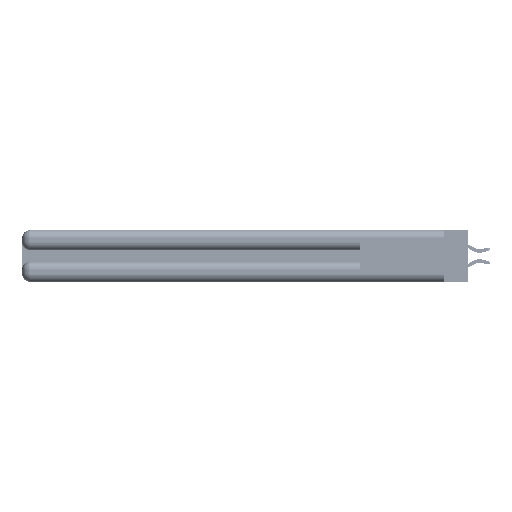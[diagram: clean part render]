
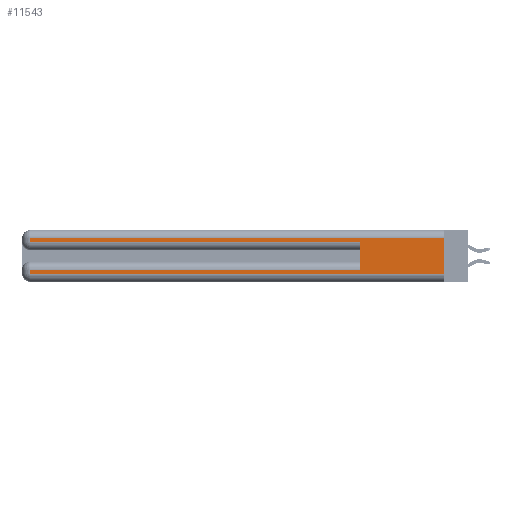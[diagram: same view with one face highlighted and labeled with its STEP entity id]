
A CAD part, left-side view. The second image highlights one B-rep face of the part: STEP entity #11543.
In plain terms, the highlighted planar face has unit normal (-1, 0, 0).
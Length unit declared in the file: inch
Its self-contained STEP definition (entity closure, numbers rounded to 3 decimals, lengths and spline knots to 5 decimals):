
#1251 = VERTEX_POINT ( 'NONE', #50723 ) ;
#2664 = ORIENTED_EDGE ( 'NONE', *, *, #31764, .T. ) ;
#2678 = CARTESIAN_POINT ( 'NONE',  ( 0., 2.94, 0.37 ) ) ;
#2749 = CARTESIAN_POINT ( 'NONE',  ( 0., 2.94, 0.06 ) ) ;
#3593 = LINE ( 'NONE', #9691, #13614 ) ;
#5487 = VECTOR ( 'NONE', #15396, 39.37008 ) ;
#5743 = VECTOR ( 'NONE', #54405, 39.37008 ) ;
#6292 = AXIS2_PLACEMENT_3D ( 'NONE', #16166, #46097, #20479 ) ;
#6643 = CARTESIAN_POINT ( 'NONE',  ( 0., 2.94, 0.31 ) ) ;
#7628 = PLANE ( 'NONE',  #6292 ) ;
#7849 = LINE ( 'NONE', #32007, #27851 ) ;
#8331 = CARTESIAN_POINT ( 'NONE',  ( 0., 0., 0.37 ) ) ;
#9218 = DIRECTION ( 'NONE',  ( 0., 1., 0. ) ) ;
#9309 = EDGE_CURVE ( 'NONE', #15465, #48542, #51947, .T. ) ;
#9337 = VECTOR ( 'NONE', #27100, 39.37008 ) ;
#9691 = CARTESIAN_POINT ( 'NONE',  ( 0., 0., 0.285 ) ) ;
#11543 = ADVANCED_FACE ( 'NONE', ( #34423 ), #7628, .F. ) ;
#12615 = CARTESIAN_POINT ( 'NONE',  ( 0., 0., 0.06 ) ) ;
#12629 = ORIENTED_EDGE ( 'NONE', *, *, #18950, .T. ) ;
#13614 = VECTOR ( 'NONE', #39954, 39.37008 ) ;
#13884 = VERTEX_POINT ( 'NONE', #6643 ) ;
#14214 = CARTESIAN_POINT ( 'NONE',  ( 0., 0., 0.31 ) ) ;
#15396 = DIRECTION ( 'NONE',  ( 0., 0., -1. ) ) ;
#15465 = VERTEX_POINT ( 'NONE', #48258 ) ;
#16166 = CARTESIAN_POINT ( 'NONE',  ( 0., 0., 0.37 ) ) ;
#16676 = ORIENTED_EDGE ( 'NONE', *, *, #44009, .T. ) ;
#17075 = LINE ( 'NONE', #45810, #5743 ) ;
#17283 = ORIENTED_EDGE ( 'NONE', *, *, #9309, .F. ) ;
#17862 = VECTOR ( 'NONE', #25252, 39.37008 ) ;
#18209 = EDGE_CURVE ( 'NONE', #24839, #1251, #7849, .T. ) ;
#18950 = EDGE_CURVE ( 'NONE', #13884, #49784, #17075, .T. ) ;
#20479 = DIRECTION ( 'NONE',  ( 0., 0., -1. ) ) ;
#23707 = CARTESIAN_POINT ( 'NONE',  ( 0., 2.94, 0.085 ) ) ;
#24839 = VERTEX_POINT ( 'NONE', #25220 ) ;
#24963 = EDGE_CURVE ( 'NONE', #24839, #52079, #31530, .T. ) ;
#25220 = CARTESIAN_POINT ( 'NONE',  ( 0., 0.6, 0.085 ) ) ;
#25252 = DIRECTION ( 'NONE',  ( 0., 0., -1. ) ) ;
#27100 = DIRECTION ( 'NONE',  ( 0., 1., 0. ) ) ;
#27337 = ORIENTED_EDGE ( 'NONE', *, *, #47613, .T. ) ;
#27851 = VECTOR ( 'NONE', #27921, 39.37008 ) ;
#27921 = DIRECTION ( 'NONE',  ( 0., 0., 1. ) ) ;
#31517 = VERTEX_POINT ( 'NONE', #2749 ) ;
#31530 = LINE ( 'NONE', #43373, #38910 ) ;
#31764 = EDGE_CURVE ( 'NONE', #31517, #48542, #52536, .T. ) ;
#32007 = CARTESIAN_POINT ( 'NONE',  ( 0., 0.6, 0.145 ) ) ;
#33362 = ORIENTED_EDGE ( 'NONE', *, *, #24963, .T. ) ;
#34423 = FACE_OUTER_BOUND ( 'NONE', #48812, .T. ) ;
#38217 = LINE ( 'NONE', #2678, #5487 ) ;
#38910 = VECTOR ( 'NONE', #9218, 39.37008 ) ;
#39954 = DIRECTION ( 'NONE',  ( 0., -1., 0. ) ) ;
#41196 = VECTOR ( 'NONE', #51326, 39.37008 ) ;
#43373 = CARTESIAN_POINT ( 'NONE',  ( 0., 0., 0.085 ) ) ;
#43419 = LINE ( 'NONE', #14214, #9337 ) ;
#44009 = EDGE_CURVE ( 'NONE', #49784, #1251, #3593, .T. ) ;
#44789 = ORIENTED_EDGE ( 'NONE', *, *, #49004, .T. ) ;
#45808 = CARTESIAN_POINT ( 'NONE',  ( 0., 2.94, 0.285 ) ) ;
#45810 = CARTESIAN_POINT ( 'NONE',  ( 0., 2.94, 0.37 ) ) ;
#46097 = DIRECTION ( 'NONE',  ( 1., 0., 0. ) ) ;
#47055 = CARTESIAN_POINT ( 'NONE',  ( 0., 0., 0.06 ) ) ;
#47613 = EDGE_CURVE ( 'NONE', #15465, #13884, #43419, .T. ) ;
#48258 = CARTESIAN_POINT ( 'NONE',  ( 0., 0., 0.31 ) ) ;
#48542 = VERTEX_POINT ( 'NONE', #12615 ) ;
#48812 = EDGE_LOOP ( 'NONE', ( #17283, #27337, #12629, #16676, #54833, #33362, #44789, #2664 ) ) ;
#49004 = EDGE_CURVE ( 'NONE', #52079, #31517, #38217, .T. ) ;
#49784 = VERTEX_POINT ( 'NONE', #45808 ) ;
#50723 = CARTESIAN_POINT ( 'NONE',  ( 0., 0.6, 0.285 ) ) ;
#51326 = DIRECTION ( 'NONE',  ( 0., -1., 0. ) ) ;
#51947 = LINE ( 'NONE', #8331, #17862 ) ;
#52079 = VERTEX_POINT ( 'NONE', #23707 ) ;
#52536 = LINE ( 'NONE', #47055, #41196 ) ;
#54405 = DIRECTION ( 'NONE',  ( 0., 0., -1. ) ) ;
#54833 = ORIENTED_EDGE ( 'NONE', *, *, #18209, .F. ) ;
